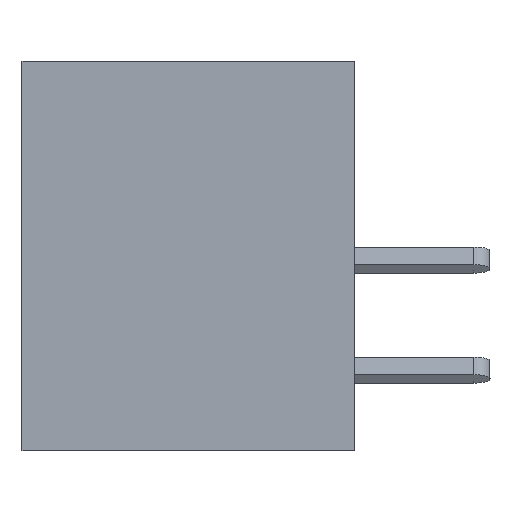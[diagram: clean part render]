
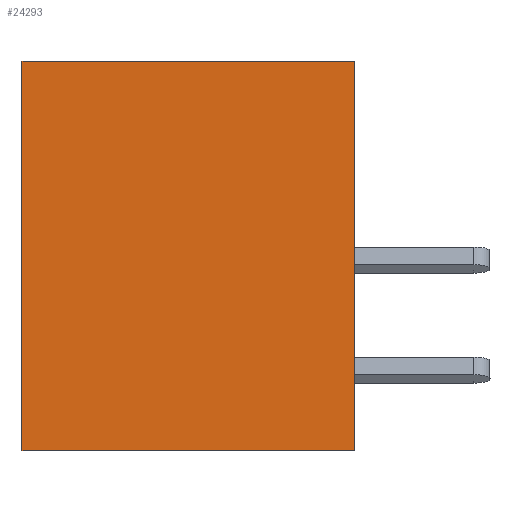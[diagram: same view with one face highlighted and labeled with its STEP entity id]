
A CAD part, left-side view. The second image highlights one B-rep face of the part: STEP entity #24293.
In plain terms, the highlighted planar face has unit normal (-1, 0, 0).
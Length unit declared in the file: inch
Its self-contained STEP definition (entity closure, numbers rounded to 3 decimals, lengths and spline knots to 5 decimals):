
#253 = CARTESIAN_POINT ( 'NONE',  ( 0., 0., -0.531 ) ) ;
#389 = PLANE ( 'NONE',  #3960 ) ;
#477 = DIRECTION ( 'NONE',  ( 0., 0., -1. ) ) ;
#3435 = ORIENTED_EDGE ( 'NONE', *, *, #24292, .F. ) ;
#3686 = VECTOR ( 'NONE', #13972, 39.37008 ) ;
#3960 = AXIS2_PLACEMENT_3D ( 'NONE', #9797, #6032, #477 ) ;
#3988 = DIRECTION ( 'NONE',  ( 0., 0., 1. ) ) ;
#4304 = CARTESIAN_POINT ( 'NONE',  ( 0., 0.453, 0. ) ) ;
#4956 = CARTESIAN_POINT ( 'NONE',  ( 0., 0., 0. ) ) ;
#5222 = LINE ( 'NONE', #7244, #19601 ) ;
#5917 = ORIENTED_EDGE ( 'NONE', *, *, #12574, .F. ) ;
#5933 = CARTESIAN_POINT ( 'NONE',  ( 0., 0.453, 0. ) ) ;
#6032 = DIRECTION ( 'NONE',  ( 1., 0., 0. ) ) ;
#7244 = CARTESIAN_POINT ( 'NONE',  ( 0., 0.453, 0. ) ) ;
#9797 = CARTESIAN_POINT ( 'NONE',  ( 0., 0.453, 0. ) ) ;
#10040 = VERTEX_POINT ( 'NONE', #5933 ) ;
#10221 = CARTESIAN_POINT ( 'NONE',  ( 0., 0., 0. ) ) ;
#10448 = EDGE_CURVE ( 'NONE', #18199, #17631, #22068, .T. ) ;
#10898 = VECTOR ( 'NONE', #3988, 39.37008 ) ;
#11629 = CARTESIAN_POINT ( 'NONE',  ( 0., 0.453, -0.531 ) ) ;
#12423 = VERTEX_POINT ( 'NONE', #4956 ) ;
#12574 = EDGE_CURVE ( 'NONE', #10040, #12423, #5222, .T. ) ;
#13641 = LINE ( 'NONE', #10221, #3686 ) ;
#13695 = EDGE_CURVE ( 'NONE', #17631, #12423, #13641, .T. ) ;
#13972 = DIRECTION ( 'NONE',  ( 0., 0., 1. ) ) ;
#16081 = FACE_OUTER_BOUND ( 'NONE', #23384, .T. ) ;
#16137 = VECTOR ( 'NONE', #21080, 39.37008 ) ;
#17631 = VERTEX_POINT ( 'NONE', #253 ) ;
#18199 = VERTEX_POINT ( 'NONE', #18549 ) ;
#18549 = CARTESIAN_POINT ( 'NONE',  ( 0., 0.453, -0.531 ) ) ;
#19601 = VECTOR ( 'NONE', #20139, 39.37008 ) ;
#19739 = LINE ( 'NONE', #4304, #10898 ) ;
#20139 = DIRECTION ( 'NONE',  ( 0., -1., 0. ) ) ;
#21080 = DIRECTION ( 'NONE',  ( 0., -1., 0. ) ) ;
#22068 = LINE ( 'NONE', #11629, #16137 ) ;
#23384 = EDGE_LOOP ( 'NONE', ( #23563, #5917, #3435, #23827 ) ) ;
#23563 = ORIENTED_EDGE ( 'NONE', *, *, #13695, .T. ) ;
#23827 = ORIENTED_EDGE ( 'NONE', *, *, #10448, .T. ) ;
#24292 = EDGE_CURVE ( 'NONE', #18199, #10040, #19739, .T. ) ;
#24293 = ADVANCED_FACE ( 'NONE', ( #16081 ), #389, .F. ) ;
